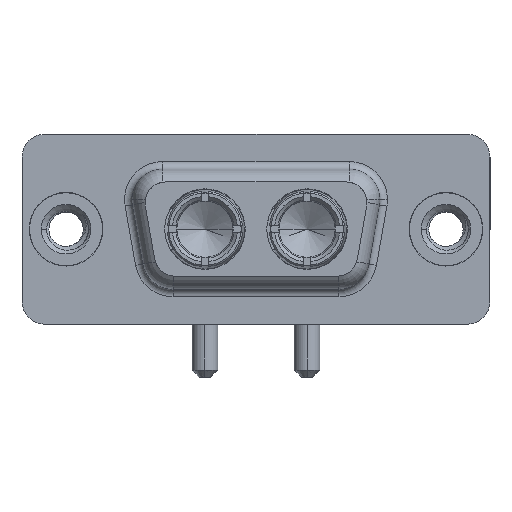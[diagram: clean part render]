
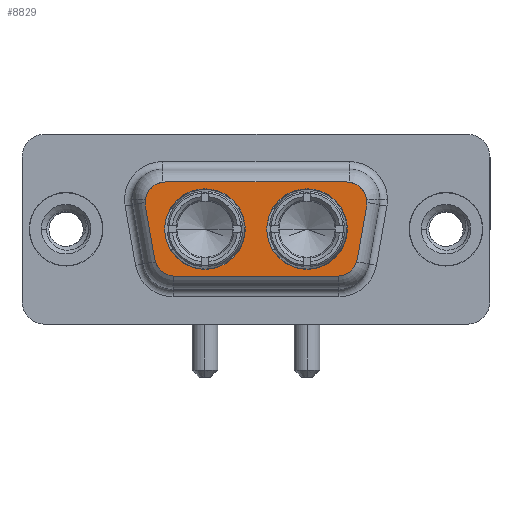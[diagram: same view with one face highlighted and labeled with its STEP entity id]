
A CAD part, top view. The second image highlights one B-rep face of the part: STEP entity #8829.
In plain terms, the highlighted planar face has unit normal (0, 0, 1).
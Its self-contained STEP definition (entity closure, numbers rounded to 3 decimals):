
#63 = DIRECTION ( 'NONE',  ( 0., 0., 1. ) ) ;
#201 = ORIENTED_EDGE ( 'NONE', *, *, #6462, .F. ) ;
#209 = CARTESIAN_POINT ( 'NONE',  ( 6.55, 1.75, 6.2 ) ) ;
#420 = CIRCLE ( 'NONE', #6520, 2.65 ) ;
#424 = VERTEX_POINT ( 'NONE', #11459 ) ;
#481 = AXIS2_PLACEMENT_3D ( 'NONE', #1105, #63, #4699 ) ;
#639 = EDGE_LOOP ( 'NONE', ( #6924, #11418, #6168, #1518, #11883, #8056, #10920, #1560, #2713 ) ) ;
#768 = DIRECTION ( 'NONE',  ( -1., 0., 0. ) ) ;
#885 = CARTESIAN_POINT ( 'NONE',  ( 18.45, 1.75, 6.2 ) ) ;
#953 = DIRECTION ( 'NONE',  ( -1., 0., 0. ) ) ;
#1009 = DIRECTION ( 'NONE',  ( 0., 0., 1. ) ) ;
#1105 = CARTESIAN_POINT ( 'NONE',  ( 15.86, 0., 6.2 ) ) ;
#1189 = EDGE_CURVE ( 'NONE', #4826, #8862, #8555, .T. ) ;
#1413 = ORIENTED_EDGE ( 'NONE', *, *, #2232, .F. ) ;
#1518 = ORIENTED_EDGE ( 'NONE', *, *, #3679, .T. ) ;
#1543 = DIRECTION ( 'NONE',  ( 0.174, -0.985, 0. ) ) ;
#1560 = ORIENTED_EDGE ( 'NONE', *, *, #8131, .T. ) ;
#1810 = CARTESIAN_POINT ( 'NONE',  ( 17.833, -1.75, 6.2 ) ) ;
#1963 = CARTESIAN_POINT ( 'NONE',  ( 19.779, 1.516, 6.2 ) ) ;
#1994 = DIRECTION ( 'NONE',  ( -1., 0., 0. ) ) ;
#2161 = CARTESIAN_POINT ( 'NONE',  ( 17.833, -3.1, 6.2 ) ) ;
#2231 = VERTEX_POINT ( 'NONE', #4165 ) ;
#2232 = EDGE_CURVE ( 'NONE', #11439, #10016, #420, .T. ) ;
#2384 = AXIS2_PLACEMENT_3D ( 'NONE', #6616, #7350, #8471 ) ;
#2417 = EDGE_LOOP ( 'NONE', ( #201, #1413 ) ) ;
#2432 = ORIENTED_EDGE ( 'NONE', *, *, #10278, .F. ) ;
#2488 = CARTESIAN_POINT ( 'NONE',  ( 5.838, -1.984, 6.2 ) ) ;
#2583 = CIRCLE ( 'NONE', #9468, 1.35 ) ;
#2709 = AXIS2_PLACEMENT_3D ( 'NONE', #2931, #6681, #1994 ) ;
#2713 = ORIENTED_EDGE ( 'NONE', *, *, #9120, .T. ) ;
#2866 = EDGE_CURVE ( 'NONE', #4952, #8305, #6125, .T. ) ;
#2931 = CARTESIAN_POINT ( 'NONE',  ( 7.167, -1.75, 6.2 ) ) ;
#3130 = VERTEX_POINT ( 'NONE', #5376 ) ;
#3358 = CARTESIAN_POINT ( 'NONE',  ( 19.162, -1.984, 6.2 ) ) ;
#3477 = CARTESIAN_POINT ( 'NONE',  ( 5.221, 1.516, 6.2 ) ) ;
#3518 = VERTEX_POINT ( 'NONE', #3358 ) ;
#3679 = EDGE_CURVE ( 'NONE', #3518, #4826, #7109, .T. ) ;
#3747 = EDGE_CURVE ( 'NONE', #8093, #3518, #8016, .T. ) ;
#3839 = EDGE_CURVE ( 'NONE', #7736, #2231, #5267, .T. ) ;
#3978 = AXIS2_PLACEMENT_3D ( 'NONE', #8545, #8477, #953 ) ;
#3991 = DIRECTION ( 'NONE',  ( 1., 0., 0. ) ) ;
#4165 = CARTESIAN_POINT ( 'NONE',  ( 7.167, -3.1, 6.2 ) ) ;
#4177 = VECTOR ( 'NONE', #1543, 1000. ) ;
#4251 = LINE ( 'NONE', #7189, #6065 ) ;
#4412 = LINE ( 'NONE', #2488, #4177 ) ;
#4541 = FACE_BOUND ( 'NONE', #8154, .T. ) ;
#4616 = DIRECTION ( 'NONE',  ( 0., 0., 1. ) ) ;
#4699 = DIRECTION ( 'NONE',  ( 1., 0., 0. ) ) ;
#4792 = CARTESIAN_POINT ( 'NONE',  ( 18.45, 3.1, 6.2 ) ) ;
#4826 = VERTEX_POINT ( 'NONE', #1963 ) ;
#4952 = VERTEX_POINT ( 'NONE', #9955 ) ;
#5267 = CIRCLE ( 'NONE', #2709, 1.35 ) ;
#5376 = CARTESIAN_POINT ( 'NONE',  ( 5.2, 1.75, 6.2 ) ) ;
#5810 = DIRECTION ( 'NONE',  ( 1., 0., 0. ) ) ;
#6065 = VECTOR ( 'NONE', #9041, 1000. ) ;
#6125 = CIRCLE ( 'NONE', #2384, 2.65 ) ;
#6168 = ORIENTED_EDGE ( 'NONE', *, *, #3747, .T. ) ;
#6201 = CARTESIAN_POINT ( 'NONE',  ( 19.779, 1.516, 6.2 ) ) ;
#6289 = EDGE_CURVE ( 'NONE', #8862, #424, #4251, .T. ) ;
#6409 = CIRCLE ( 'NONE', #481, 2.65 ) ;
#6462 = EDGE_CURVE ( 'NONE', #10016, #11439, #10954, .T. ) ;
#6520 = AXIS2_PLACEMENT_3D ( 'NONE', #8612, #11690, #8733 ) ;
#6599 = EDGE_CURVE ( 'NONE', #424, #3130, #9378, .T. ) ;
#6616 = CARTESIAN_POINT ( 'NONE',  ( 15.86, 0., 6.2 ) ) ;
#6681 = DIRECTION ( 'NONE',  ( 0., 0., 1. ) ) ;
#6740 = FACE_OUTER_BOUND ( 'NONE', #639, .T. ) ;
#6902 = LINE ( 'NONE', #8824, #11036 ) ;
#6924 = ORIENTED_EDGE ( 'NONE', *, *, #3839, .T. ) ;
#7109 = LINE ( 'NONE', #6201, #10962 ) ;
#7189 = CARTESIAN_POINT ( 'NONE',  ( 6.55, 3.1, 6.2 ) ) ;
#7321 = VERTEX_POINT ( 'NONE', #3477 ) ;
#7350 = DIRECTION ( 'NONE',  ( 0., 0., 1. ) ) ;
#7353 = AXIS2_PLACEMENT_3D ( 'NONE', #885, #11995, #11314 ) ;
#7407 = AXIS2_PLACEMENT_3D ( 'NONE', #9281, #4616, #12142 ) ;
#7736 = VERTEX_POINT ( 'NONE', #7902 ) ;
#7902 = CARTESIAN_POINT ( 'NONE',  ( 5.838, -1.984, 6.2 ) ) ;
#8016 = CIRCLE ( 'NONE', #10168, 1.35 ) ;
#8056 = ORIENTED_EDGE ( 'NONE', *, *, #6289, .T. ) ;
#8093 = VERTEX_POINT ( 'NONE', #2161 ) ;
#8131 = EDGE_CURVE ( 'NONE', #3130, #7321, #2583, .T. ) ;
#8154 = EDGE_LOOP ( 'NONE', ( #11312, #2432 ) ) ;
#8161 = EDGE_CURVE ( 'NONE', #2231, #8093, #6902, .T. ) ;
#8305 = VERTEX_POINT ( 'NONE', #9173 ) ;
#8471 = DIRECTION ( 'NONE',  ( 1., 0., 0. ) ) ;
#8477 = DIRECTION ( 'NONE',  ( 0., 0., -1. ) ) ;
#8545 = CARTESIAN_POINT ( 'NONE',  ( 7.167, -1.75, 6.2 ) ) ;
#8555 = CIRCLE ( 'NONE', #7353, 1.35 ) ;
#8612 = CARTESIAN_POINT ( 'NONE',  ( 9.14, 0., 6.2 ) ) ;
#8704 = CARTESIAN_POINT ( 'NONE',  ( 6.55, 1.75, 6.2 ) ) ;
#8733 = DIRECTION ( 'NONE',  ( 1., 0., 0. ) ) ;
#8766 = DIRECTION ( 'NONE',  ( 0., 0., 1. ) ) ;
#8824 = CARTESIAN_POINT ( 'NONE',  ( 17.833, -3.1, 6.2 ) ) ;
#8829 = ADVANCED_FACE ( 'NONE', ( #4541, #12062, #6740 ), #11319, .F. ) ;
#8862 = VERTEX_POINT ( 'NONE', #4792 ) ;
#9041 = DIRECTION ( 'NONE',  ( -1., 0., 0. ) ) ;
#9120 = EDGE_CURVE ( 'NONE', #7321, #7736, #4412, .T. ) ;
#9173 = CARTESIAN_POINT ( 'NONE',  ( 13.21, 0., 6.2 ) ) ;
#9281 = CARTESIAN_POINT ( 'NONE',  ( 9.14, 0., 6.2 ) ) ;
#9321 = CARTESIAN_POINT ( 'NONE',  ( 6.49, 0., 6.2 ) ) ;
#9378 = CIRCLE ( 'NONE', #10560, 1.35 ) ;
#9468 = AXIS2_PLACEMENT_3D ( 'NONE', #8704, #8766, #5810 ) ;
#9736 = DIRECTION ( 'NONE',  ( 1., 0., 0. ) ) ;
#9940 = DIRECTION ( 'NONE',  ( 0.174, 0.985, 0. ) ) ;
#9955 = CARTESIAN_POINT ( 'NONE',  ( 18.51, 0., 6.2 ) ) ;
#10016 = VERTEX_POINT ( 'NONE', #11726 ) ;
#10168 = AXIS2_PLACEMENT_3D ( 'NONE', #1810, #1009, #768 ) ;
#10278 = EDGE_CURVE ( 'NONE', #8305, #4952, #6409, .T. ) ;
#10560 = AXIS2_PLACEMENT_3D ( 'NONE', #209, #11509, #3991 ) ;
#10920 = ORIENTED_EDGE ( 'NONE', *, *, #6599, .T. ) ;
#10954 = CIRCLE ( 'NONE', #7407, 2.65 ) ;
#10962 = VECTOR ( 'NONE', #9940, 1000. ) ;
#11036 = VECTOR ( 'NONE', #9736, 1000. ) ;
#11312 = ORIENTED_EDGE ( 'NONE', *, *, #2866, .F. ) ;
#11314 = DIRECTION ( 'NONE',  ( -1., 0., 0. ) ) ;
#11319 = PLANE ( 'NONE',  #3978 ) ;
#11418 = ORIENTED_EDGE ( 'NONE', *, *, #8161, .T. ) ;
#11439 = VERTEX_POINT ( 'NONE', #9321 ) ;
#11459 = CARTESIAN_POINT ( 'NONE',  ( 6.55, 3.1, 6.2 ) ) ;
#11509 = DIRECTION ( 'NONE',  ( 0., 0., 1. ) ) ;
#11690 = DIRECTION ( 'NONE',  ( 0., 0., 1. ) ) ;
#11726 = CARTESIAN_POINT ( 'NONE',  ( 11.79, 0., 6.2 ) ) ;
#11883 = ORIENTED_EDGE ( 'NONE', *, *, #1189, .T. ) ;
#11995 = DIRECTION ( 'NONE',  ( 0., 0., 1. ) ) ;
#12062 = FACE_BOUND ( 'NONE', #2417, .T. ) ;
#12142 = DIRECTION ( 'NONE',  ( 1., 0., 0. ) ) ;
